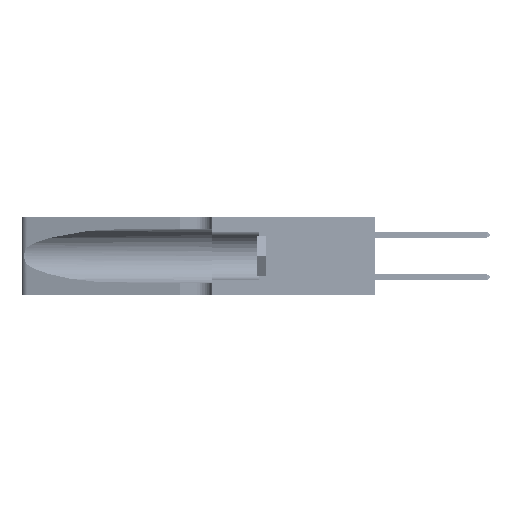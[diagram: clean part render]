
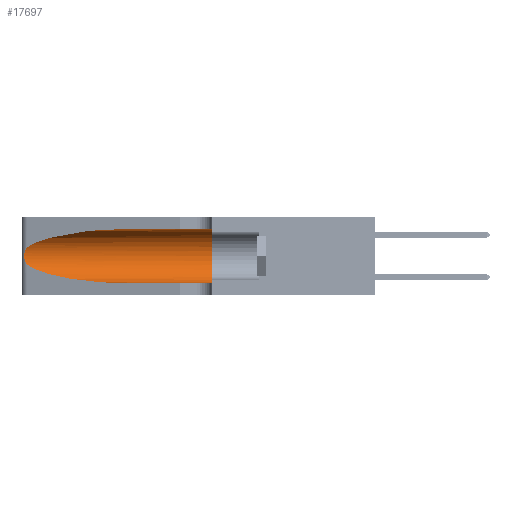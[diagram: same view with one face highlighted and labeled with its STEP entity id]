
A CAD part, left-side view. The second image highlights one B-rep face of the part: STEP entity #17697.
In plain terms, the highlighted cylindrical face has radius 3.308 mm (diameter 6.617 mm), a partial arc.
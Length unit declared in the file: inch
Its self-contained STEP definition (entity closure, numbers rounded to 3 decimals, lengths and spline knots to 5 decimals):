
#205 = DIRECTION ( 'NONE',  ( 0., 1., 0. ) ) ;
#1880 = FACE_OUTER_BOUND ( 'NONE', #47450, .T. ) ;
#2012 = CARTESIAN_POINT ( 'NONE',  ( 0.18966, 0.96281, 0.05475 ) ) ;
#2840 = CARTESIAN_POINT ( 'NONE',  ( 0.1305, 1.61858, 0.185 ) ) ;
#2975 = CARTESIAN_POINT ( 'NONE',  ( 0.25555, 1.22993, 0.14849 ) ) ;
#3546 = DIRECTION ( 'NONE',  ( 0., 0., -1. ) ) ;
#6707 = AXIS2_PLACEMENT_3D ( 'NONE', #2840, #35759, #3546 ) ;
#6742 = CARTESIAN_POINT ( 'NONE',  ( 0.25787, 1.23484, 0.2124 ) ) ;
#6940 = CARTESIAN_POINT ( 'NONE',  ( 0.1305, 0.72297, 0.31525 ) ) ;
#7080 = CARTESIAN_POINT ( 'NONE',  ( 0.25639, 1.23184, 0.21858 ) ) ;
#8178 = CARTESIAN_POINT ( 'NONE',  ( 0.1305, 0.35, 0.05475 ) ) ;
#10403 = VERTEX_POINT ( 'NONE', #16788 ) ;
#10819 = CARTESIAN_POINT ( 'NONE',  ( 0.25856, 1.23593, 0.16098 ) ) ;
#10997 = CARTESIAN_POINT ( 'NONE',  ( 0.25789, 1.23486, 0.15765 ) ) ;
#11167 = CARTESIAN_POINT ( 'NONE',  ( 0.25555, 1.22994, 0.2215 ) ) ;
#12826 = CARTESIAN_POINT ( 'NONE',  ( 0.25487, 1.22718, 0.22369 ) ) ;
#13349 = ORIENTED_EDGE ( 'NONE', *, *, #22962, .F. ) ;
#13440 = VECTOR ( 'NONE', #31903, 39.37008 ) ;
#14739 = EDGE_CURVE ( 'NONE', #10403, #46418, #41680, .T. ) ;
#15133 = CARTESIAN_POINT ( 'NONE',  ( 0.18966, 0.96281, 0.31525 ) ) ;
#15267 = CARTESIAN_POINT ( 'NONE',  ( 0.25639, 1.23186, 0.15144 ) ) ;
#15683 = EDGE_CURVE ( 'NONE', #32540, #31636, #34498, .T. ) ;
#16744 = ORIENTED_EDGE ( 'NONE', *, *, #15683, .T. ) ;
#16788 = CARTESIAN_POINT ( 'NONE',  ( 0.1305, 0.35, 0.31525 ) ) ;
#17120 = CARTESIAN_POINT ( 'NONE',  ( 0.1305, 1.61858, 0.31525 ) ) ;
#17697 = ADVANCED_FACE ( 'NONE', ( #1880 ), #20992, .F. ) ;
#18353 = ORIENTED_EDGE ( 'NONE', *, *, #20059, .T. ) ;
#18665 = CARTESIAN_POINT ( 'NONE',  ( 0.26075, 1.23896, 0.19203 ) ) ;
#19187 = CARTESIAN_POINT ( 'NONE',  ( 0.25487, 1.22718, 0.22369 ) ) ;
#20059 = EDGE_CURVE ( 'NONE', #31636, #50715, #51262, .T. ) ;
#20992 = CYLINDRICAL_SURFACE ( 'NONE', #6707, 0.13025 ) ;
#21677 = LINE ( 'NONE', #40647, #13440 ) ;
#22903 = CARTESIAN_POINT ( 'NONE',  ( 0.26018, 1.23835, 0.19895 ) ) ;
#22962 = EDGE_CURVE ( 'NONE', #50982, #10403, #51343, .T. ) ;
#23201 = ORIENTED_EDGE ( 'NONE', *, *, #25244, .T. ) ;
#23294 = CARTESIAN_POINT ( 'NONE',  ( 0.25487, 1.22718, 0.22369 ) ) ;
#25244 = EDGE_CURVE ( 'NONE', #50982, #32540, #32174, .T. ) ;
#25649 = CARTESIAN_POINT ( 'NONE',  ( 0.1305, 0.72297, 0.05475 ) ) ;
#26221 = CARTESIAN_POINT ( 'NONE',  ( 0.2373, 1.15595, 0.08982 ) ) ;
#27690 = VECTOR ( 'NONE', #45618, 39.37008 ) ;
#30663 = CARTESIAN_POINT ( 'NONE',  ( 0.1305, 0.72297, 0.05475 ) ) ;
#31636 = VERTEX_POINT ( 'NONE', #32511 ) ;
#31903 = DIRECTION ( 'NONE',  ( 0., -1., 0. ) ) ;
#32174 =( BOUNDED_CURVE ( )  B_SPLINE_CURVE ( 3, ( #6940, #15133, #35413, #23294 ),
 .UNSPECIFIED., .F., .T. ) 
 B_SPLINE_CURVE_WITH_KNOTS ( ( 4, 4 ),
 ( 1.5708, 2.84003 ),
 .UNSPECIFIED. ) 
 CURVE ( )  GEOMETRIC_REPRESENTATION_ITEM ( )  RATIONAL_B_SPLINE_CURVE ( ( 1., 0.87, 0.87, 1. ) ) 
 REPRESENTATION_ITEM ( '' )  );
#32511 = CARTESIAN_POINT ( 'NONE',  ( 0.25487, 1.22718, 0.14631 ) ) ;
#32540 = VERTEX_POINT ( 'NONE', #12826 ) ;
#34498 = B_SPLINE_CURVE_WITH_KNOTS ( 'NONE', 3,
 ( #19187, #11167, #7080, #6742, #38944, #22903, #18665, #51844, #47682, #10819, #10997, #15267, #2975, #51299 ),
 .UNSPECIFIED., .F., .F.,
 ( 4, 2, 2, 2, 2, 2, 4 ),
 ( 0., 0.00027, 0.00053, 0.00107, 0.0016, 0.00187, 0.00214 ),
 .UNSPECIFIED. ) ;
#35413 = CARTESIAN_POINT ( 'NONE',  ( 0.2373, 1.15595, 0.28018 ) ) ;
#35759 = DIRECTION ( 'NONE',  ( 0., -1., 0. ) ) ;
#38678 = CARTESIAN_POINT ( 'NONE',  ( 0.25487, 1.22718, 0.14631 ) ) ;
#38944 = CARTESIAN_POINT ( 'NONE',  ( 0.25854, 1.2359, 0.20912 ) ) ;
#40647 = CARTESIAN_POINT ( 'NONE',  ( 0.1305, 1.61858, 0.05475 ) ) ;
#41680 = CIRCLE ( 'NONE', #52389, 0.13025 ) ;
#42335 = CARTESIAN_POINT ( 'NONE',  ( 0.1305, 0.72297, 0.31525 ) ) ;
#44365 = DIRECTION ( 'NONE',  ( 0., 0., 1. ) ) ;
#44915 = CARTESIAN_POINT ( 'NONE',  ( 0.1305, 0.35, 0.185 ) ) ;
#45618 = DIRECTION ( 'NONE',  ( 0., -1., 0. ) ) ;
#45668 = EDGE_CURVE ( 'NONE', #50715, #46418, #21677, .T. ) ;
#46418 = VERTEX_POINT ( 'NONE', #8178 ) ;
#47450 = EDGE_LOOP ( 'NONE', ( #23201, #16744, #18353, #51692, #52661, #13349 ) ) ;
#47682 = CARTESIAN_POINT ( 'NONE',  ( 0.26017, 1.23833, 0.17102 ) ) ;
#50715 = VERTEX_POINT ( 'NONE', #25649 ) ;
#50982 = VERTEX_POINT ( 'NONE', #42335 ) ;
#51262 =( BOUNDED_CURVE ( )  B_SPLINE_CURVE ( 3, ( #38678, #26221, #2012, #30663 ),
 .UNSPECIFIED., .F., .F. ) 
 B_SPLINE_CURVE_WITH_KNOTS ( ( 4, 4 ),
 ( 3.44316, 4.71239 ),
 .UNSPECIFIED. ) 
 CURVE ( )  GEOMETRIC_REPRESENTATION_ITEM ( )  RATIONAL_B_SPLINE_CURVE ( ( 1., 0.87, 0.87, 1. ) ) 
 REPRESENTATION_ITEM ( '' )  );
#51299 = CARTESIAN_POINT ( 'NONE',  ( 0.25487, 1.22718, 0.14631 ) ) ;
#51343 = LINE ( 'NONE', #17120, #27690 ) ;
#51692 = ORIENTED_EDGE ( 'NONE', *, *, #45668, .T. ) ;
#51844 = CARTESIAN_POINT ( 'NONE',  ( 0.26075, 1.23896, 0.178 ) ) ;
#52389 = AXIS2_PLACEMENT_3D ( 'NONE', #44915, #205, #44365 ) ;
#52661 = ORIENTED_EDGE ( 'NONE', *, *, #14739, .F. ) ;
